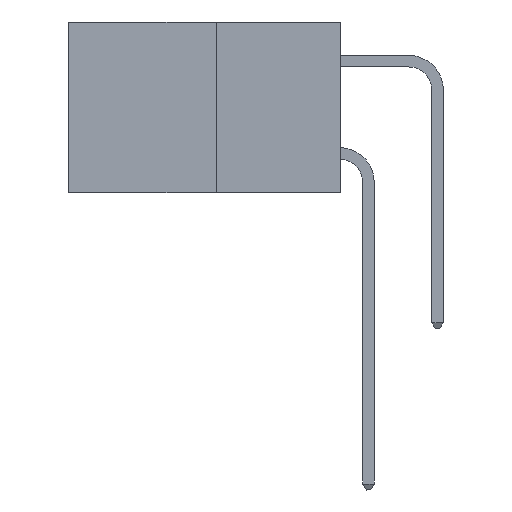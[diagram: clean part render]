
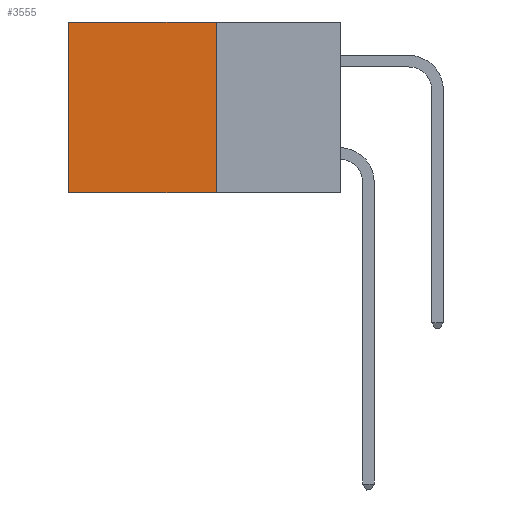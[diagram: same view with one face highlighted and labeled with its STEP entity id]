
A CAD part, left-side view. The second image highlights one B-rep face of the part: STEP entity #3555.
In plain terms, the highlighted planar face has unit normal (-1, 0, 0).
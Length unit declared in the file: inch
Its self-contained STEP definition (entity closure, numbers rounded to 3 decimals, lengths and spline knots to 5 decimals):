
#62 = PLANE ( 'NONE',  #19282 ) ;
#83 = CARTESIAN_POINT ( 'NONE',  ( 0.277, 0.27, -0.37 ) ) ;
#1015 = CARTESIAN_POINT ( 'NONE',  ( 0.277, 0.27, -0.37 ) ) ;
#1399 = DIRECTION ( 'NONE',  ( 0., 1., 0. ) ) ;
#1649 = LINE ( 'NONE', #3505, #10496 ) ;
#1950 = CARTESIAN_POINT ( 'NONE',  ( 0.277, 0.27, 0. ) ) ;
#2491 = DIRECTION ( 'NONE',  ( 0., 0., -1. ) ) ;
#2623 = LINE ( 'NONE', #10431, #6757 ) ;
#3250 = EDGE_CURVE ( 'NONE', #10696, #6985, #22615, .T. ) ;
#3438 = ORIENTED_EDGE ( 'NONE', *, *, #21564, .T. ) ;
#3505 = CARTESIAN_POINT ( 'NONE',  ( 0.277, 0.27, -0.37 ) ) ;
#3555 = ADVANCED_FACE ( 'NONE', ( #15378 ), #62, .F. ) ;
#4057 = VECTOR ( 'NONE', #1399, 39.37008 ) ;
#4524 = EDGE_CURVE ( 'NONE', #17578, #21479, #2623, .T. ) ;
#5289 = DIRECTION ( 'NONE',  ( 0., 0., -1. ) ) ;
#5456 = CARTESIAN_POINT ( 'NONE',  ( 0.277, 0.27, 0. ) ) ;
#6757 = VECTOR ( 'NONE', #12211, 39.37008 ) ;
#6985 = VERTEX_POINT ( 'NONE', #9476 ) ;
#9476 = CARTESIAN_POINT ( 'NONE',  ( 0.277, 0.59, 0. ) ) ;
#9919 = ORIENTED_EDGE ( 'NONE', *, *, #17260, .F. ) ;
#9982 = CARTESIAN_POINT ( 'NONE',  ( 0.277, 0.59, -0.37 ) ) ;
#10431 = CARTESIAN_POINT ( 'NONE',  ( 0.277, 0.27, -0.37 ) ) ;
#10496 = VECTOR ( 'NONE', #5289, 39.37008 ) ;
#10696 = VERTEX_POINT ( 'NONE', #5456 ) ;
#11556 = ORIENTED_EDGE ( 'NONE', *, *, #3250, .T. ) ;
#11753 = DIRECTION ( 'NONE',  ( 0., 0., -1. ) ) ;
#12211 = DIRECTION ( 'NONE',  ( 0., 1., 0. ) ) ;
#12540 = VECTOR ( 'NONE', #11753, 39.37008 ) ;
#12541 = EDGE_LOOP ( 'NONE', ( #3438, #17906, #9919, #11556 ) ) ;
#15378 = FACE_OUTER_BOUND ( 'NONE', #12541, .T. ) ;
#16773 = CARTESIAN_POINT ( 'NONE',  ( 0.277, 0.59, -0.37 ) ) ;
#17260 = EDGE_CURVE ( 'NONE', #10696, #17578, #1649, .T. ) ;
#17578 = VERTEX_POINT ( 'NONE', #1015 ) ;
#17718 = LINE ( 'NONE', #9982, #12540 ) ;
#17906 = ORIENTED_EDGE ( 'NONE', *, *, #4524, .F. ) ;
#19282 = AXIS2_PLACEMENT_3D ( 'NONE', #83, #22500, #2491 ) ;
#21479 = VERTEX_POINT ( 'NONE', #16773 ) ;
#21564 = EDGE_CURVE ( 'NONE', #6985, #21479, #17718, .T. ) ;
#22500 = DIRECTION ( 'NONE',  ( 1., 0., 0. ) ) ;
#22615 = LINE ( 'NONE', #1950, #4057 ) ;
